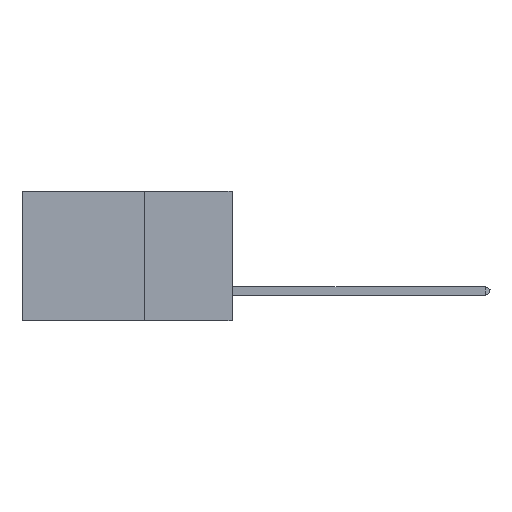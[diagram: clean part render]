
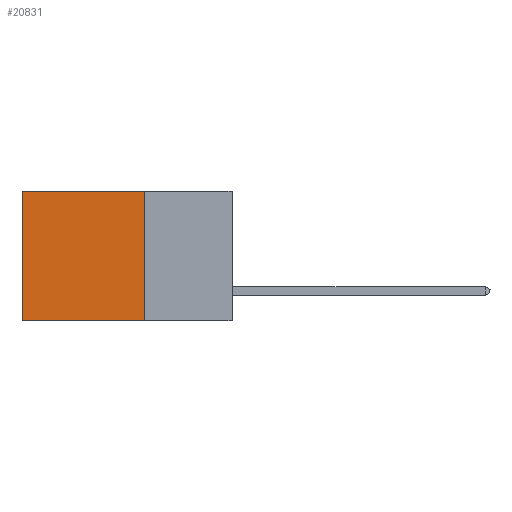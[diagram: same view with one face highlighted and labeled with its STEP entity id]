
A CAD part, left-side view. The second image highlights one B-rep face of the part: STEP entity #20831.
In plain terms, the highlighted planar face has unit normal (-1, 0, 0).
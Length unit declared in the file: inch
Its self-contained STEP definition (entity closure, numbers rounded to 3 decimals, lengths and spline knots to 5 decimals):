
#2343 = CARTESIAN_POINT ( 'NONE',  ( 0.2875, 0.6, 0. ) ) ;
#2998 = CARTESIAN_POINT ( 'NONE',  ( 0.2875, 0.25, 0. ) ) ;
#4585 = LINE ( 'NONE', #2343, #9319 ) ;
#5740 = DIRECTION ( 'NONE',  ( 0., 1., 0. ) ) ;
#5945 = ORIENTED_EDGE ( 'NONE', *, *, #7375, .T. ) ;
#6379 = DIRECTION ( 'NONE',  ( 0., 0., -1. ) ) ;
#6883 = CARTESIAN_POINT ( 'NONE',  ( 0.2875, 0.25, 0. ) ) ;
#7375 = EDGE_CURVE ( 'NONE', #24295, #25925, #8306, .T. ) ;
#8306 = LINE ( 'NONE', #2998, #14011 ) ;
#9048 = DIRECTION ( 'NONE',  ( 1., 0., 0. ) ) ;
#9319 = VECTOR ( 'NONE', #21725, 39.37008 ) ;
#10208 = ORIENTED_EDGE ( 'NONE', *, *, #16508, .F. ) ;
#10589 = CARTESIAN_POINT ( 'NONE',  ( 0.2875, 0.25, -0.37 ) ) ;
#10824 = EDGE_LOOP ( 'NONE', ( #15605, #10208, #14764, #5945 ) ) ;
#14011 = VECTOR ( 'NONE', #5740, 39.37008 ) ;
#14764 = ORIENTED_EDGE ( 'NONE', *, *, #24186, .F. ) ;
#14946 = PLANE ( 'NONE',  #34579 ) ;
#14983 = LINE ( 'NONE', #15476, #16814 ) ;
#15476 = CARTESIAN_POINT ( 'NONE',  ( 0.2875, 0.25, -0.37 ) ) ;
#15605 = ORIENTED_EDGE ( 'NONE', *, *, #22825, .T. ) ;
#15640 = DIRECTION ( 'NONE',  ( 0., 0., -1. ) ) ;
#16508 = EDGE_CURVE ( 'NONE', #33798, #16936, #14983, .T. ) ;
#16814 = VECTOR ( 'NONE', #26793, 39.37008 ) ;
#16936 = VERTEX_POINT ( 'NONE', #26728 ) ;
#20831 = ADVANCED_FACE ( 'NONE', ( #32062 ), #14946, .F. ) ;
#21725 = DIRECTION ( 'NONE',  ( 0., 0., -1. ) ) ;
#22825 = EDGE_CURVE ( 'NONE', #25925, #16936, #4585, .T. ) ;
#23781 = LINE ( 'NONE', #28617, #26394 ) ;
#24186 = EDGE_CURVE ( 'NONE', #24295, #33798, #23781, .T. ) ;
#24295 = VERTEX_POINT ( 'NONE', #6883 ) ;
#25900 = CARTESIAN_POINT ( 'NONE',  ( 0.2875, 0.25, 0. ) ) ;
#25925 = VERTEX_POINT ( 'NONE', #26225 ) ;
#26225 = CARTESIAN_POINT ( 'NONE',  ( 0.2875, 0.6, 0. ) ) ;
#26394 = VECTOR ( 'NONE', #15640, 39.37008 ) ;
#26728 = CARTESIAN_POINT ( 'NONE',  ( 0.2875, 0.6, -0.37 ) ) ;
#26793 = DIRECTION ( 'NONE',  ( 0., 1., 0. ) ) ;
#28617 = CARTESIAN_POINT ( 'NONE',  ( 0.2875, 0.25, 0. ) ) ;
#32062 = FACE_OUTER_BOUND ( 'NONE', #10824, .T. ) ;
#33798 = VERTEX_POINT ( 'NONE', #10589 ) ;
#34579 = AXIS2_PLACEMENT_3D ( 'NONE', #25900, #9048, #6379 ) ;
